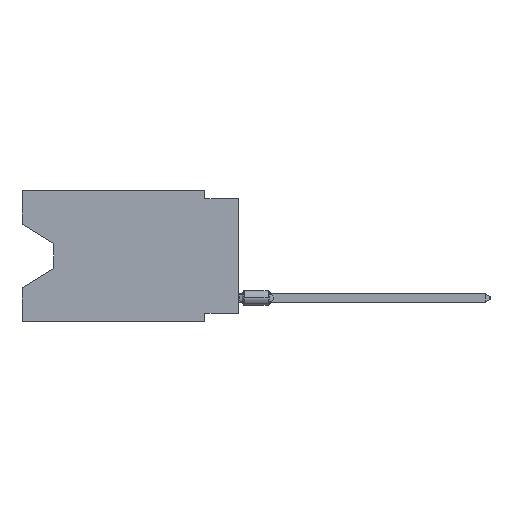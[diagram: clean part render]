
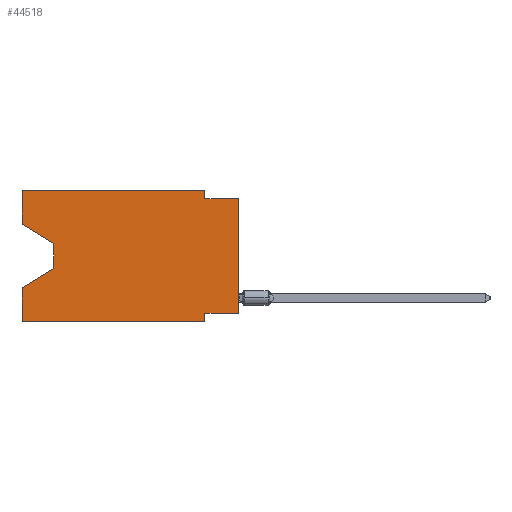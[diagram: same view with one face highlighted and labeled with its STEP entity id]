
A CAD part, left-side view. The second image highlights one B-rep face of the part: STEP entity #44518.
In plain terms, the highlighted planar face has unit normal (-1, 0, 0).
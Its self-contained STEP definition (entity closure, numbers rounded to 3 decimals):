
#1544 = CARTESIAN_POINT ( 'NONE',  ( 0., 16.383, 0. ) ) ;
#1777 = LINE ( 'NONE', #16804, #48668 ) ;
#4769 = CARTESIAN_POINT ( 'NONE',  ( 0., 16.383, 0. ) ) ;
#4804 = VERTEX_POINT ( 'NONE', #8679 ) ;
#4972 = EDGE_CURVE ( 'NONE', #15335, #10799, #14766, .T. ) ;
#5313 = CARTESIAN_POINT ( 'NONE',  ( 0., 2.54, 0. ) ) ;
#5509 = EDGE_CURVE ( 'NONE', #18043, #55176, #38655, .T. ) ;
#6808 = CARTESIAN_POINT ( 'NONE',  ( 0., 13.97, -5.893 ) ) ;
#6999 = ORIENTED_EDGE ( 'NONE', *, *, #15008, .F. ) ;
#8391 = VECTOR ( 'NONE', #36873, 1000. ) ;
#8679 = CARTESIAN_POINT ( 'NONE',  ( 0., 0., -0.635 ) ) ;
#9127 = VECTOR ( 'NONE', #52073, 1000. ) ;
#9433 = EDGE_LOOP ( 'NONE', ( #26778, #32278, #67441, #46839, #41180, #30205, #6999, #13949, #62952, #48884, #67707, #41192 ) ) ;
#10799 = VERTEX_POINT ( 'NONE', #52826 ) ;
#11653 = VECTOR ( 'NONE', #27164, 1000. ) ;
#12598 = EDGE_CURVE ( 'NONE', #36764, #14533, #59170, .T. ) ;
#13001 = CARTESIAN_POINT ( 'NONE',  ( 0., 0., -0.635 ) ) ;
#13949 = ORIENTED_EDGE ( 'NONE', *, *, #25416, .T. ) ;
#14533 = VERTEX_POINT ( 'NONE', #48381 ) ;
#14766 = LINE ( 'NONE', #30813, #9127 ) ;
#14970 = PLANE ( 'NONE',  #64743 ) ;
#15008 = EDGE_CURVE ( 'NONE', #37875, #58314, #54222, .T. ) ;
#15335 = VERTEX_POINT ( 'NONE', #5313 ) ;
#15659 = FACE_OUTER_BOUND ( 'NONE', #9433, .T. ) ;
#16804 = CARTESIAN_POINT ( 'NONE',  ( 0., 13.97, -5.893 ) ) ;
#18043 = VERTEX_POINT ( 'NONE', #49114 ) ;
#18065 = VECTOR ( 'NONE', #37037, 1000. ) ;
#18158 = VECTOR ( 'NONE', #33425, 1000. ) ;
#18497 = DIRECTION ( 'NONE',  ( 0., 0., 1. ) ) ;
#21031 = EDGE_CURVE ( 'NONE', #24674, #14533, #1777, .T. ) ;
#21183 = LINE ( 'NONE', #58812, #44438 ) ;
#21660 = VECTOR ( 'NONE', #48369, 1000. ) ;
#23474 = LINE ( 'NONE', #13001, #53685 ) ;
#24674 = VERTEX_POINT ( 'NONE', #6808 ) ;
#25416 = EDGE_CURVE ( 'NONE', #37875, #4804, #44318, .T. ) ;
#26778 = ORIENTED_EDGE ( 'NONE', *, *, #5509, .T. ) ;
#27164 = DIRECTION ( 'NONE',  ( 0., 0., -1. ) ) ;
#28375 = DIRECTION ( 'NONE',  ( 0., 0., 1. ) ) ;
#30205 = ORIENTED_EDGE ( 'NONE', *, *, #32323, .F. ) ;
#30813 = CARTESIAN_POINT ( 'NONE',  ( 0., 2.54, 0. ) ) ;
#31421 = VERTEX_POINT ( 'NONE', #64354 ) ;
#31816 = CARTESIAN_POINT ( 'NONE',  ( 0., 16.383, -9.906 ) ) ;
#32278 = ORIENTED_EDGE ( 'NONE', *, *, #41465, .T. ) ;
#32323 = EDGE_CURVE ( 'NONE', #58314, #63940, #21183, .T. ) ;
#32353 = CARTESIAN_POINT ( 'NONE',  ( 0., 16.383, 0. ) ) ;
#33425 = DIRECTION ( 'NONE',  ( 0., -0.855, -0.519 ) ) ;
#34290 = DIRECTION ( 'NONE',  ( 0., -1., 0. ) ) ;
#36764 = VERTEX_POINT ( 'NONE', #67468 ) ;
#36873 = DIRECTION ( 'NONE',  ( 0., -1., 0. ) ) ;
#36947 = CARTESIAN_POINT ( 'NONE',  ( 0., 16.383, 0. ) ) ;
#37037 = DIRECTION ( 'NONE',  ( 0., -1., 0. ) ) ;
#37639 = CARTESIAN_POINT ( 'NONE',  ( 0., 13.97, -4.013 ) ) ;
#37875 = VERTEX_POINT ( 'NONE', #51181 ) ;
#38205 = VECTOR ( 'NONE', #28375, 1000. ) ;
#38210 = CARTESIAN_POINT ( 'NONE',  ( 0., 0., -9.271 ) ) ;
#38325 = CARTESIAN_POINT ( 'NONE',  ( 0., 16.383, -2.546 ) ) ;
#38655 = LINE ( 'NONE', #38325, #18158 ) ;
#39229 = DIRECTION ( 'NONE',  ( 0., 1., 0. ) ) ;
#39730 = EDGE_CURVE ( 'NONE', #18043, #31421, #64664, .T. ) ;
#41180 = ORIENTED_EDGE ( 'NONE', *, *, #45228, .T. ) ;
#41192 = ORIENTED_EDGE ( 'NONE', *, *, #39730, .F. ) ;
#41465 = EDGE_CURVE ( 'NONE', #55176, #24674, #48787, .T. ) ;
#42092 = DIRECTION ( 'NONE',  ( 0., 0., -1. ) ) ;
#42447 = LINE ( 'NONE', #4769, #8391 ) ;
#42522 = DIRECTION ( 'NONE',  ( 0., 0., -1. ) ) ;
#44318 = LINE ( 'NONE', #50210, #53366 ) ;
#44438 = VECTOR ( 'NONE', #42092, 1000. ) ;
#44518 = ADVANCED_FACE ( 'NONE', ( #15659 ), #14970, .F. ) ;
#45228 = EDGE_CURVE ( 'NONE', #36764, #63940, #58990, .T. ) ;
#45550 = CARTESIAN_POINT ( 'NONE',  ( 0., 2.54, -9.906 ) ) ;
#45762 = EDGE_CURVE ( 'NONE', #10799, #4804, #23474, .T. ) ;
#46839 = ORIENTED_EDGE ( 'NONE', *, *, #12598, .F. ) ;
#48369 = DIRECTION ( 'NONE',  ( 0., 0., 1. ) ) ;
#48381 = CARTESIAN_POINT ( 'NONE',  ( 0., 16.383, -7.36 ) ) ;
#48668 = VECTOR ( 'NONE', #54443, 1000. ) ;
#48787 = LINE ( 'NONE', #37639, #11653 ) ;
#48884 = ORIENTED_EDGE ( 'NONE', *, *, #4972, .F. ) ;
#49114 = CARTESIAN_POINT ( 'NONE',  ( 0., 16.383, -2.546 ) ) ;
#50210 = CARTESIAN_POINT ( 'NONE',  ( 0., 0., 0. ) ) ;
#50870 = CARTESIAN_POINT ( 'NONE',  ( 0., 2.54, -9.271 ) ) ;
#51181 = CARTESIAN_POINT ( 'NONE',  ( 0., 0., -9.271 ) ) ;
#52073 = DIRECTION ( 'NONE',  ( 0., 0., -1. ) ) ;
#52826 = CARTESIAN_POINT ( 'NONE',  ( 0., 2.54, -0.635 ) ) ;
#53366 = VECTOR ( 'NONE', #18497, 1000. ) ;
#53685 = VECTOR ( 'NONE', #34290, 1000. ) ;
#54222 = LINE ( 'NONE', #38210, #68605 ) ;
#54443 = DIRECTION ( 'NONE',  ( 0., 0.855, -0.519 ) ) ;
#55176 = VERTEX_POINT ( 'NONE', #58674 ) ;
#58189 = DIRECTION ( 'NONE',  ( 1., 0., 0. ) ) ;
#58314 = VERTEX_POINT ( 'NONE', #50870 ) ;
#58674 = CARTESIAN_POINT ( 'NONE',  ( 0., 13.97, -4.013 ) ) ;
#58812 = CARTESIAN_POINT ( 'NONE',  ( 0., 2.54, -9.906 ) ) ;
#58990 = LINE ( 'NONE', #31816, #18065 ) ;
#59170 = LINE ( 'NONE', #32353, #21660 ) ;
#62562 = EDGE_CURVE ( 'NONE', #31421, #15335, #42447, .T. ) ;
#62952 = ORIENTED_EDGE ( 'NONE', *, *, #45762, .F. ) ;
#63940 = VERTEX_POINT ( 'NONE', #45550 ) ;
#64354 = CARTESIAN_POINT ( 'NONE',  ( 0., 16.383, 0. ) ) ;
#64664 = LINE ( 'NONE', #1544, #38205 ) ;
#64743 = AXIS2_PLACEMENT_3D ( 'NONE', #36947, #58189, #42522 ) ;
#67441 = ORIENTED_EDGE ( 'NONE', *, *, #21031, .T. ) ;
#67468 = CARTESIAN_POINT ( 'NONE',  ( 0., 16.383, -9.906 ) ) ;
#67707 = ORIENTED_EDGE ( 'NONE', *, *, #62562, .F. ) ;
#68605 = VECTOR ( 'NONE', #39229, 1000. ) ;
